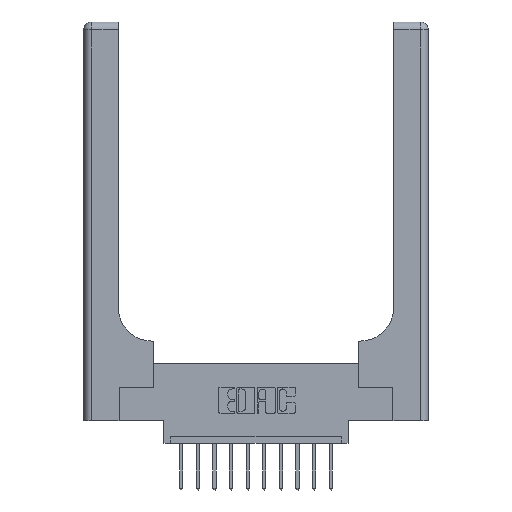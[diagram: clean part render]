
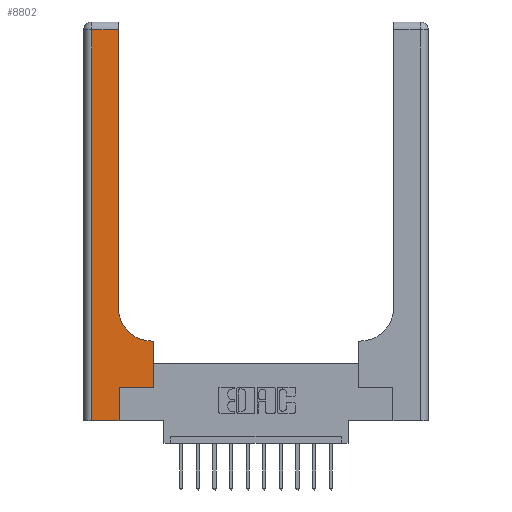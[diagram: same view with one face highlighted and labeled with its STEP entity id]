
A CAD part, top view. The second image highlights one B-rep face of the part: STEP entity #8802.
In plain terms, the highlighted planar face has unit normal (0, 0, 1).
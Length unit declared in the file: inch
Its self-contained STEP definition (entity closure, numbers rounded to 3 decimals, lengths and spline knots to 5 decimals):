
#26 = CARTESIAN_POINT ( 'NONE',  ( 0.51, 0.6, 0.37 ) ) ;
#443 = EDGE_CURVE ( 'NONE', #9641, #7570, #5361, .T. ) ;
#728 = CARTESIAN_POINT ( 'NONE',  ( 0.06, 3., 0.37 ) ) ;
#785 = EDGE_CURVE ( 'NONE', #3902, #4987, #5942, .T. ) ;
#1184 = CARTESIAN_POINT ( 'NONE',  ( 0., 2.94, 0.37 ) ) ;
#1226 = DIRECTION ( 'NONE',  ( 0., 1., 0. ) ) ;
#1334 = CARTESIAN_POINT ( 'NONE',  ( 0.06, 2.94, 0.37 ) ) ;
#1340 = CARTESIAN_POINT ( 'NONE',  ( 0.265, 0., 0.37 ) ) ;
#1671 = VECTOR ( 'NONE', #2851, 39.37008 ) ;
#1696 = CARTESIAN_POINT ( 'NONE',  ( 0.528, 0.6, 0.37 ) ) ;
#2104 = AXIS2_PLACEMENT_3D ( 'NONE', #6126, #14639, #9421 ) ;
#2374 = CARTESIAN_POINT ( 'NONE',  ( 0.26, 3., 0.37 ) ) ;
#2399 = VECTOR ( 'NONE', #7603, 39.37008 ) ;
#2430 = CARTESIAN_POINT ( 'NONE',  ( 0.265, 0.25, 0.37 ) ) ;
#2851 = DIRECTION ( 'NONE',  ( 1., 0., 0. ) ) ;
#2940 = PLANE ( 'NONE',  #9212 ) ;
#3436 = ORIENTED_EDGE ( 'NONE', *, *, #443, .T. ) ;
#3730 = ORIENTED_EDGE ( 'NONE', *, *, #13648, .T. ) ;
#3902 = VERTEX_POINT ( 'NONE', #1696 ) ;
#4110 = ORIENTED_EDGE ( 'NONE', *, *, #15356, .T. ) ;
#4306 = VERTEX_POINT ( 'NONE', #5586 ) ;
#4432 = EDGE_CURVE ( 'NONE', #7842, #8681, #10726, .T. ) ;
#4909 = VECTOR ( 'NONE', #11838, 39.37008 ) ;
#4987 = VERTEX_POINT ( 'NONE', #26 ) ;
#4998 = CARTESIAN_POINT ( 'NONE',  ( 0.528, 0.25, 0.37 ) ) ;
#5195 = EDGE_CURVE ( 'NONE', #7570, #8279, #12789, .T. ) ;
#5361 = LINE ( 'NONE', #6517, #1671 ) ;
#5368 = ORIENTED_EDGE ( 'NONE', *, *, #4432, .T. ) ;
#5413 = VERTEX_POINT ( 'NONE', #4998 ) ;
#5470 = ORIENTED_EDGE ( 'NONE', *, *, #5950, .T. ) ;
#5586 = CARTESIAN_POINT ( 'NONE',  ( 0.26, 0.85, 0.37 ) ) ;
#5622 = VECTOR ( 'NONE', #1226, 39.37008 ) ;
#5623 = ORIENTED_EDGE ( 'NONE', *, *, #785, .T. ) ;
#5807 = CARTESIAN_POINT ( 'NONE',  ( 0.06, 0., 0.37 ) ) ;
#5942 = LINE ( 'NONE', #8062, #11740 ) ;
#5950 = EDGE_CURVE ( 'NONE', #8681, #9641, #6046, .T. ) ;
#6046 = LINE ( 'NONE', #728, #4909 ) ;
#6126 = CARTESIAN_POINT ( 'NONE',  ( 0.51, 0.85, 0.37 ) ) ;
#6386 = DIRECTION ( 'NONE',  ( -1., 0., 0. ) ) ;
#6441 = CARTESIAN_POINT ( 'NONE',  ( 0., 3., 0.37 ) ) ;
#6454 = LINE ( 'NONE', #7317, #11458 ) ;
#6517 = CARTESIAN_POINT ( 'NONE',  ( 0., 0., 0.37 ) ) ;
#6805 = CARTESIAN_POINT ( 'NONE',  ( 0.265, 0.25, 0.37 ) ) ;
#7011 = EDGE_LOOP ( 'NONE', ( #12099, #5368, #5470, #3436, #14513, #12471, #3730, #5623, #4110 ) ) ;
#7317 = CARTESIAN_POINT ( 'NONE',  ( 0.528, 0.25, 0.37 ) ) ;
#7365 = EDGE_CURVE ( 'NONE', #4306, #7842, #14577, .T. ) ;
#7401 = VECTOR ( 'NONE', #12155, 39.37008 ) ;
#7570 = VERTEX_POINT ( 'NONE', #1340 ) ;
#7603 = DIRECTION ( 'NONE',  ( 0., 1., 0. ) ) ;
#7842 = VERTEX_POINT ( 'NONE', #15284 ) ;
#8062 = CARTESIAN_POINT ( 'NONE',  ( 0.26, 0.6, 0.37 ) ) ;
#8279 = VERTEX_POINT ( 'NONE', #6805 ) ;
#8681 = VERTEX_POINT ( 'NONE', #1334 ) ;
#8802 = ADVANCED_FACE ( 'NONE', ( #13415 ), #2940, .F. ) ;
#9212 = AXIS2_PLACEMENT_3D ( 'NONE', #6441, #12778, #6386 ) ;
#9421 = DIRECTION ( 'NONE',  ( 1., 0., 0. ) ) ;
#9470 = EDGE_CURVE ( 'NONE', #8279, #5413, #14703, .T. ) ;
#9641 = VERTEX_POINT ( 'NONE', #5807 ) ;
#9769 = VECTOR ( 'NONE', #13580, 39.37008 ) ;
#10726 = LINE ( 'NONE', #1184, #7401 ) ;
#11458 = VECTOR ( 'NONE', #15733, 39.37008 ) ;
#11708 = DIRECTION ( 'NONE',  ( -1., 0., 0. ) ) ;
#11740 = VECTOR ( 'NONE', #11708, 39.37008 ) ;
#11838 = DIRECTION ( 'NONE',  ( 0., -1., 0. ) ) ;
#12099 = ORIENTED_EDGE ( 'NONE', *, *, #7365, .T. ) ;
#12155 = DIRECTION ( 'NONE',  ( -1., 0., 0. ) ) ;
#12471 = ORIENTED_EDGE ( 'NONE', *, *, #9470, .T. ) ;
#12633 = CARTESIAN_POINT ( 'NONE',  ( 0.265, 0., 0.37 ) ) ;
#12778 = DIRECTION ( 'NONE',  ( 0., 0., -1. ) ) ;
#12789 = LINE ( 'NONE', #12633, #2399 ) ;
#13415 = FACE_OUTER_BOUND ( 'NONE', #7011, .T. ) ;
#13580 = DIRECTION ( 'NONE',  ( 1., 0., 0. ) ) ;
#13648 = EDGE_CURVE ( 'NONE', #5413, #3902, #6454, .T. ) ;
#14214 = CIRCLE ( 'NONE', #2104, 0.25 ) ;
#14513 = ORIENTED_EDGE ( 'NONE', *, *, #5195, .T. ) ;
#14577 = LINE ( 'NONE', #2374, #5622 ) ;
#14639 = DIRECTION ( 'NONE',  ( 0., 0., -1. ) ) ;
#14703 = LINE ( 'NONE', #2430, #9769 ) ;
#15284 = CARTESIAN_POINT ( 'NONE',  ( 0.26, 2.94, 0.37 ) ) ;
#15356 = EDGE_CURVE ( 'NONE', #4987, #4306, #14214, .T. ) ;
#15733 = DIRECTION ( 'NONE',  ( 0., 1., 0. ) ) ;
